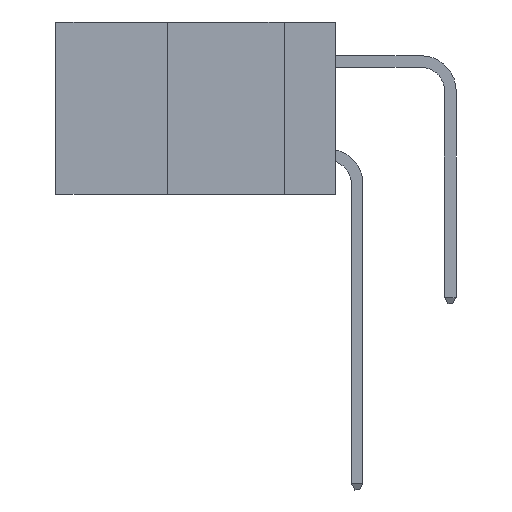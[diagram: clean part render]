
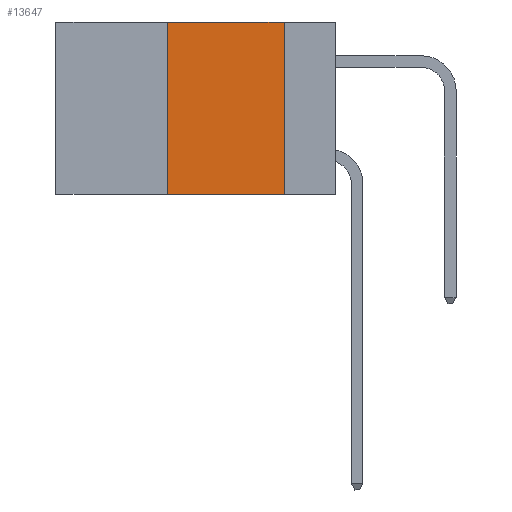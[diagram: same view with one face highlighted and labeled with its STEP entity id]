
A CAD part, left-side view. The second image highlights one B-rep face of the part: STEP entity #13647.
In plain terms, the highlighted planar face has unit normal (-1, 0, 0).
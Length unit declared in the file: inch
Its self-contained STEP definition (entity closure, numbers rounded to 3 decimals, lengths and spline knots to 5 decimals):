
#798 = CARTESIAN_POINT ( 'NONE',  ( 0., 0.11, 0. ) ) ;
#906 = DIRECTION ( 'NONE',  ( 1., 0., 0. ) ) ;
#1111 = LINE ( 'NONE', #16463, #20546 ) ;
#1278 = VERTEX_POINT ( 'NONE', #28098 ) ;
#2521 = ORIENTED_EDGE ( 'NONE', *, *, #20051, .T. ) ;
#2906 = EDGE_CURVE ( 'NONE', #21433, #10824, #29582, .T. ) ;
#4439 = VECTOR ( 'NONE', #18853, 39.37008 ) ;
#4508 = FACE_OUTER_BOUND ( 'NONE', #18811, .T. ) ;
#4975 = VERTEX_POINT ( 'NONE', #11862 ) ;
#5793 = DIRECTION ( 'NONE',  ( 0., -1., 0. ) ) ;
#6157 = VECTOR ( 'NONE', #18410, 39.37008 ) ;
#6967 = ORIENTED_EDGE ( 'NONE', *, *, #29139, .F. ) ;
#8709 = EDGE_CURVE ( 'NONE', #1278, #4975, #1111, .T. ) ;
#10824 = VERTEX_POINT ( 'NONE', #27274 ) ;
#11862 = CARTESIAN_POINT ( 'NONE',  ( 0., 0.36, 0. ) ) ;
#12837 = LINE ( 'NONE', #25960, #6157 ) ;
#12839 = ORIENTED_EDGE ( 'NONE', *, *, #2906, .F. ) ;
#13647 = ADVANCED_FACE ( 'NONE', ( #4508 ), #28633, .F. ) ;
#16463 = CARTESIAN_POINT ( 'NONE',  ( 0., 0.36, 0. ) ) ;
#18349 = CARTESIAN_POINT ( 'NONE',  ( 0., 0.6, -0.37 ) ) ;
#18410 = DIRECTION ( 'NONE',  ( 0., -1., 0. ) ) ;
#18596 = CARTESIAN_POINT ( 'NONE',  ( 0., 0.6, 0. ) ) ;
#18705 = DIRECTION ( 'NONE',  ( 0., 0., -1. ) ) ;
#18811 = EDGE_LOOP ( 'NONE', ( #12839, #6967, #21122, #2521 ) ) ;
#18853 = DIRECTION ( 'NONE',  ( 0., 0., -1. ) ) ;
#20051 = EDGE_CURVE ( 'NONE', #1278, #10824, #21071, .T. ) ;
#20546 = VECTOR ( 'NONE', #28937, 39.37008 ) ;
#21071 = LINE ( 'NONE', #18349, #27711 ) ;
#21122 = ORIENTED_EDGE ( 'NONE', *, *, #8709, .F. ) ;
#21433 = VERTEX_POINT ( 'NONE', #798 ) ;
#23665 = AXIS2_PLACEMENT_3D ( 'NONE', #18596, #906, #18705 ) ;
#23879 = CARTESIAN_POINT ( 'NONE',  ( 0., 0.11, 0. ) ) ;
#25960 = CARTESIAN_POINT ( 'NONE',  ( 0., 0.6, 0. ) ) ;
#27274 = CARTESIAN_POINT ( 'NONE',  ( 0., 0.11, -0.37 ) ) ;
#27711 = VECTOR ( 'NONE', #5793, 39.37008 ) ;
#28098 = CARTESIAN_POINT ( 'NONE',  ( 0., 0.36, -0.37 ) ) ;
#28633 = PLANE ( 'NONE',  #23665 ) ;
#28937 = DIRECTION ( 'NONE',  ( 0., 0., 1. ) ) ;
#29139 = EDGE_CURVE ( 'NONE', #4975, #21433, #12837, .T. ) ;
#29582 = LINE ( 'NONE', #23879, #4439 ) ;
